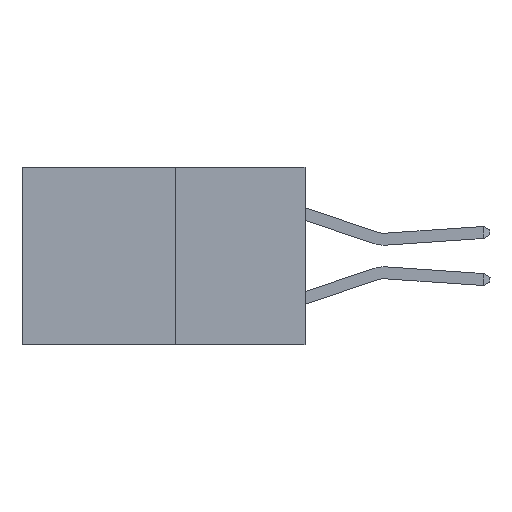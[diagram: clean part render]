
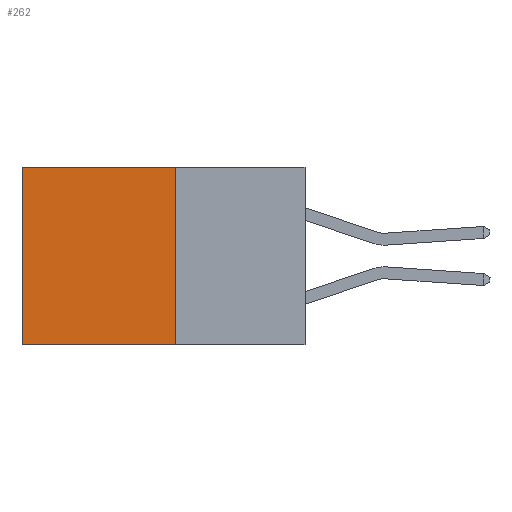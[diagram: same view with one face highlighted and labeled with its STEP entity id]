
A CAD part, left-side view. The second image highlights one B-rep face of the part: STEP entity #262.
In plain terms, the highlighted planar face has unit normal (-1, 0, 0).
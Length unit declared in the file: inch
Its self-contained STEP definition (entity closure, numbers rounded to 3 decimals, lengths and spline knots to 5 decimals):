
#14 = CARTESIAN_POINT ( 'NONE',  ( 0.277, 0.27, -0.37 ) ) ;
#262 = ADVANCED_FACE ( 'NONE', ( #2206 ), #11648, .F. ) ;
#1796 = DIRECTION ( 'NONE',  ( 0., 0., -1. ) ) ;
#1861 = EDGE_CURVE ( 'NONE', #3088, #18521, #10521, .T. ) ;
#2206 = FACE_OUTER_BOUND ( 'NONE', #8108, .T. ) ;
#3088 = VERTEX_POINT ( 'NONE', #27936 ) ;
#3788 = LINE ( 'NONE', #12043, #19495 ) ;
#4870 = LINE ( 'NONE', #30608, #29305 ) ;
#4992 = ORIENTED_EDGE ( 'NONE', *, *, #1861, .F. ) ;
#5060 = AXIS2_PLACEMENT_3D ( 'NONE', #11654, #22130, #12910 ) ;
#6550 = VERTEX_POINT ( 'NONE', #15360 ) ;
#7284 = VERTEX_POINT ( 'NONE', #28448 ) ;
#8108 = EDGE_LOOP ( 'NONE', ( #12336, #9583, #4992, #29014 ) ) ;
#9583 = ORIENTED_EDGE ( 'NONE', *, *, #19732, .F. ) ;
#9719 = CARTESIAN_POINT ( 'NONE',  ( 0.277, 0.27, -0.37 ) ) ;
#9721 = VECTOR ( 'NONE', #1796, 39.37008 ) ;
#9960 = CARTESIAN_POINT ( 'NONE',  ( 0.277, 0.59, -0.37 ) ) ;
#10521 = LINE ( 'NONE', #9719, #9721 ) ;
#11648 = PLANE ( 'NONE',  #5060 ) ;
#11654 = CARTESIAN_POINT ( 'NONE',  ( 0.277, 0.27, -0.37 ) ) ;
#12043 = CARTESIAN_POINT ( 'NONE',  ( 0.277, 0.27, 0. ) ) ;
#12336 = ORIENTED_EDGE ( 'NONE', *, *, #21524, .T. ) ;
#12543 = DIRECTION ( 'NONE',  ( 0., 0., -1. ) ) ;
#12910 = DIRECTION ( 'NONE',  ( 0., 0., -1. ) ) ;
#13081 = DIRECTION ( 'NONE',  ( 0., 1., 0. ) ) ;
#14546 = DIRECTION ( 'NONE',  ( 0., 1., 0. ) ) ;
#15027 = VECTOR ( 'NONE', #12543, 39.37008 ) ;
#15360 = CARTESIAN_POINT ( 'NONE',  ( 0.277, 0.59, 0. ) ) ;
#17668 = EDGE_CURVE ( 'NONE', #3088, #6550, #3788, .T. ) ;
#18521 = VERTEX_POINT ( 'NONE', #14 ) ;
#19495 = VECTOR ( 'NONE', #14546, 39.37008 ) ;
#19732 = EDGE_CURVE ( 'NONE', #18521, #7284, #4870, .T. ) ;
#21524 = EDGE_CURVE ( 'NONE', #6550, #7284, #22505, .T. ) ;
#22130 = DIRECTION ( 'NONE',  ( 1., 0., 0. ) ) ;
#22505 = LINE ( 'NONE', #9960, #15027 ) ;
#27936 = CARTESIAN_POINT ( 'NONE',  ( 0.277, 0.27, 0. ) ) ;
#28448 = CARTESIAN_POINT ( 'NONE',  ( 0.277, 0.59, -0.37 ) ) ;
#29014 = ORIENTED_EDGE ( 'NONE', *, *, #17668, .T. ) ;
#29305 = VECTOR ( 'NONE', #13081, 39.37008 ) ;
#30608 = CARTESIAN_POINT ( 'NONE',  ( 0.277, 0.27, -0.37 ) ) ;
